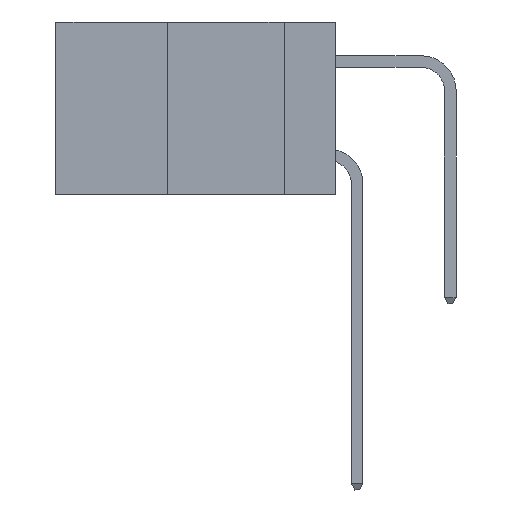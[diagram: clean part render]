
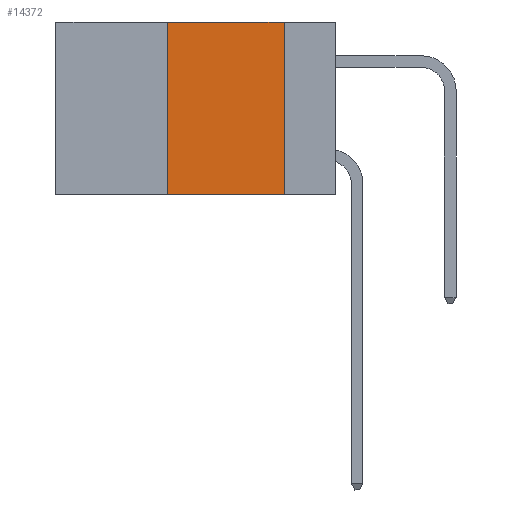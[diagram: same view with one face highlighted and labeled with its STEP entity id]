
A CAD part, left-side view. The second image highlights one B-rep face of the part: STEP entity #14372.
In plain terms, the highlighted planar face has unit normal (-1, 0, 0).
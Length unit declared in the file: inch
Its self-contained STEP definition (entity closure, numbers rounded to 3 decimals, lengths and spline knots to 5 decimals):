
#16 = AXIS2_PLACEMENT_3D ( 'NONE', #22723, #32931, #27775 ) ;
#1967 = VECTOR ( 'NONE', #33599, 39.37008 ) ;
#2767 = EDGE_CURVE ( 'NONE', #32590, #20207, #33151, .T. ) ;
#4649 = EDGE_CURVE ( 'NONE', #20207, #5799, #21285, .T. ) ;
#5799 = VERTEX_POINT ( 'NONE', #27455 ) ;
#8471 = EDGE_LOOP ( 'NONE', ( #25837, #15641, #9002, #10241 ) ) ;
#9002 = ORIENTED_EDGE ( 'NONE', *, *, #11172, .F. ) ;
#10241 = ORIENTED_EDGE ( 'NONE', *, *, #18537, .T. ) ;
#10511 = CARTESIAN_POINT ( 'NONE',  ( 0., 0.6, 0. ) ) ;
#11172 = EDGE_CURVE ( 'NONE', #31749, #32590, #21658, .T. ) ;
#13729 = CARTESIAN_POINT ( 'NONE',  ( 0., 0.11, 0. ) ) ;
#14372 = ADVANCED_FACE ( 'NONE', ( #32291 ), #36963, .F. ) ;
#15641 = ORIENTED_EDGE ( 'NONE', *, *, #2767, .F. ) ;
#18176 = LINE ( 'NONE', #36589, #1967 ) ;
#18537 = EDGE_CURVE ( 'NONE', #31749, #5799, #18176, .T. ) ;
#19532 = DIRECTION ( 'NONE',  ( 0., 0., 1. ) ) ;
#20207 = VERTEX_POINT ( 'NONE', #13729 ) ;
#20796 = VECTOR ( 'NONE', #33653, 39.37008 ) ;
#21285 = LINE ( 'NONE', #24884, #20796 ) ;
#21658 = LINE ( 'NONE', #25066, #26190 ) ;
#21912 = DIRECTION ( 'NONE',  ( 0., -1., 0. ) ) ;
#22723 = CARTESIAN_POINT ( 'NONE',  ( 0., 0.6, 0. ) ) ;
#22761 = VECTOR ( 'NONE', #21912, 39.37008 ) ;
#24884 = CARTESIAN_POINT ( 'NONE',  ( 0., 0.11, 0. ) ) ;
#25066 = CARTESIAN_POINT ( 'NONE',  ( 0., 0.36, 0. ) ) ;
#25837 = ORIENTED_EDGE ( 'NONE', *, *, #4649, .F. ) ;
#26190 = VECTOR ( 'NONE', #19532, 39.37008 ) ;
#27455 = CARTESIAN_POINT ( 'NONE',  ( 0., 0.11, -0.37 ) ) ;
#27775 = DIRECTION ( 'NONE',  ( 0., 0., -1. ) ) ;
#31749 = VERTEX_POINT ( 'NONE', #32910 ) ;
#32291 = FACE_OUTER_BOUND ( 'NONE', #8471, .T. ) ;
#32590 = VERTEX_POINT ( 'NONE', #35981 ) ;
#32910 = CARTESIAN_POINT ( 'NONE',  ( 0., 0.36, -0.37 ) ) ;
#32931 = DIRECTION ( 'NONE',  ( 1., 0., 0. ) ) ;
#33151 = LINE ( 'NONE', #10511, #22761 ) ;
#33599 = DIRECTION ( 'NONE',  ( 0., -1., 0. ) ) ;
#33653 = DIRECTION ( 'NONE',  ( 0., 0., -1. ) ) ;
#35981 = CARTESIAN_POINT ( 'NONE',  ( 0., 0.36, 0. ) ) ;
#36589 = CARTESIAN_POINT ( 'NONE',  ( 0., 0.6, -0.37 ) ) ;
#36963 = PLANE ( 'NONE',  #16 ) ;
